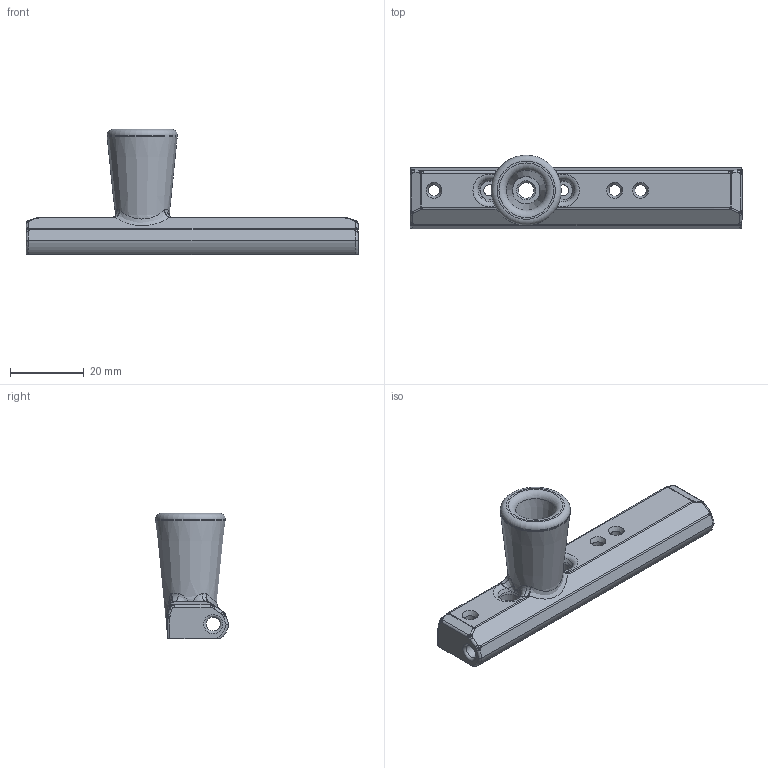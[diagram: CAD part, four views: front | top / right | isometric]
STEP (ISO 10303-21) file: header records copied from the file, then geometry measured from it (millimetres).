
FILE_DESCRIPTION(/* description */ (''),/* implementation_level */ '2;1');
FILE_NAME(/* name */ 'ARK Chargin'' Handle/Handle.step',/* time_stamp */ '2022-02-02T21:15:49-07:00',/* author */ (''),/* organization */ (''),/* preprocessor_version */ 'ST-DEVELOPER v18.1',/* originating_system */ 'Autodesk Translation Framework v10.13.0.1454',/* authorisation */ '');
FILE_SCHEMA (('AUTOMOTIVE_DESIGN { 1 0 10303 214 3 1 1 }'));
Length unit declared in the file: millimetre
Products named in the file (2): Jelly's ARK 2; GuidedHandle
Assembly tree (1 placements, depth 2):
  Jelly's ARK 2
    GuidedHandle
Bounding box: 90 x 19.92 x 34 mm (x, y, z)
Volume: 14866.6 mm3; surface area: 8458.5 mm2
Topology: 1 solids, 1 shells, 203 faces, 513 edges, 306 vertices
Faces by surface type: bspline 101, cylinder 36, plane 31, torus 19, cone 16
Full cylindrical faces by diameter (mm): 3 x2, 3.1 x3, 3.75 x1, 4.2 x1, 5 x2, 6 x1, 7.4 x1, 19 x1
Entity records: 9522 total; most frequent: CARTESIAN_POINT 4969, ORIENTED_EDGE 1010, DIRECTION 839, EDGE_CURVE 505, AXIS2_PLACEMENT_3D 365, VERTEX_POINT 306, CIRCLE 257, EDGE_LOOP 219
